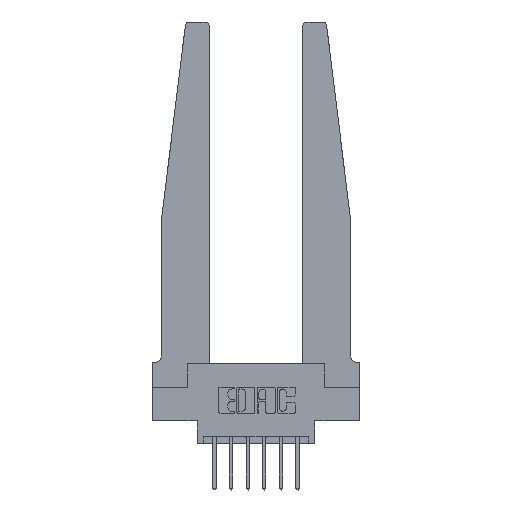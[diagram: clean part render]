
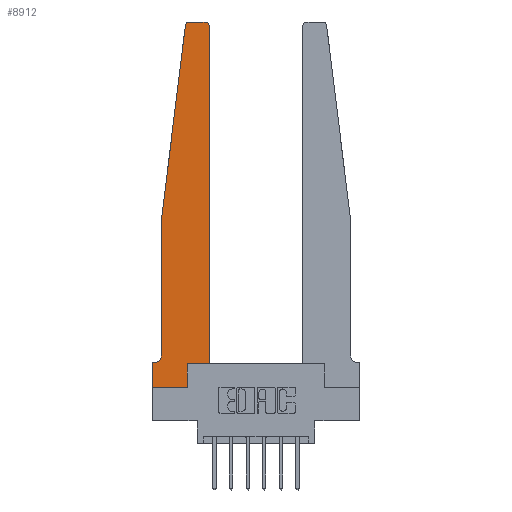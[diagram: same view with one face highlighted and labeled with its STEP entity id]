
A CAD part, top view. The second image highlights one B-rep face of the part: STEP entity #8912.
In plain terms, the highlighted planar face has unit normal (0, 0, 1).
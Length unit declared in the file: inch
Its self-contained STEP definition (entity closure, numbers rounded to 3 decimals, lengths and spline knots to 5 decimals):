
#233 = CARTESIAN_POINT ( 'NONE',  ( 0.27653, 2.72, 0.37 ) ) ;
#350 = AXIS2_PLACEMENT_3D ( 'NONE', #6943, #617, #8035 ) ;
#370 = ORIENTED_EDGE ( 'NONE', *, *, #1534, .T. ) ;
#470 = DIRECTION ( 'NONE',  ( 1., 0., 0. ) ) ;
#531 = VECTOR ( 'NONE', #470, 39.37008 ) ;
#533 = VERTEX_POINT ( 'NONE', #2530 ) ;
#617 = DIRECTION ( 'NONE',  ( 0., 0., 1. ) ) ;
#885 = LINE ( 'NONE', #7896, #531 ) ;
#1322 = DIRECTION ( 'NONE',  ( 1., 0., 0. ) ) ;
#1493 = VECTOR ( 'NONE', #3000, 39.37008 ) ;
#1534 = EDGE_CURVE ( 'NONE', #13502, #2419, #11196, .T. ) ;
#1874 = LINE ( 'NONE', #3142, #2214 ) ;
#1982 = CARTESIAN_POINT ( 'NONE',  ( 0.065, 1.25, 0.37 ) ) ;
#2042 = VERTEX_POINT ( 'NONE', #1982 ) ;
#2214 = VECTOR ( 'NONE', #5263, 39.37008 ) ;
#2419 = VERTEX_POINT ( 'NONE', #2809 ) ;
#2530 = CARTESIAN_POINT ( 'NONE',  ( 0., 0., 0.37 ) ) ;
#2577 = ORIENTED_EDGE ( 'NONE', *, *, #4362, .T. ) ;
#2700 = EDGE_CURVE ( 'NONE', #8825, #11561, #4251, .T. ) ;
#2713 = CARTESIAN_POINT ( 'NONE',  ( 0., 0., 0.37 ) ) ;
#2779 = ORIENTED_EDGE ( 'NONE', *, *, #11386, .T. ) ;
#2809 = CARTESIAN_POINT ( 'NONE',  ( 0.425, 2.72, 0.37 ) ) ;
#3000 = DIRECTION ( 'NONE',  ( 0., -1., 0. ) ) ;
#3011 = VECTOR ( 'NONE', #9632, 39.37008 ) ;
#3061 = ORIENTED_EDGE ( 'NONE', *, *, #11150, .T. ) ;
#3142 = CARTESIAN_POINT ( 'NONE',  ( 0.25, 2.75, 0.37 ) ) ;
#3811 = CARTESIAN_POINT ( 'NONE',  ( 0.2605, 0.18, 0.37 ) ) ;
#3930 = CARTESIAN_POINT ( 'NONE',  ( 0.395, 2.75, 0.37 ) ) ;
#4018 = EDGE_CURVE ( 'NONE', #4080, #13502, #885, .T. ) ;
#4080 = VERTEX_POINT ( 'NONE', #3811 ) ;
#4125 = FACE_OUTER_BOUND ( 'NONE', #7262, .T. ) ;
#4251 = CIRCLE ( 'NONE', #10601, 0.05 ) ;
#4277 = DIRECTION ( 'NONE',  ( 0., 1., 0. ) ) ;
#4280 = DIRECTION ( 'NONE',  ( -1., 0., 0. ) ) ;
#4308 = ORIENTED_EDGE ( 'NONE', *, *, #7747, .T. ) ;
#4355 = LINE ( 'NONE', #12104, #12741 ) ;
#4362 = EDGE_CURVE ( 'NONE', #4863, #12184, #1874, .T. ) ;
#4521 = DIRECTION ( 'NONE',  ( 0., 0., -1. ) ) ;
#4762 = DIRECTION ( 'NONE',  ( 0., 1., 0. ) ) ;
#4863 = VERTEX_POINT ( 'NONE', #3930 ) ;
#5131 = VECTOR ( 'NONE', #11581, 39.37008 ) ;
#5263 = DIRECTION ( 'NONE',  ( -1., 0., 0. ) ) ;
#5359 = EDGE_CURVE ( 'NONE', #5531, #4080, #4355, .T. ) ;
#5436 = CARTESIAN_POINT ( 'NONE',  ( 0.395, 2.72, 0.37 ) ) ;
#5531 = VERTEX_POINT ( 'NONE', #10488 ) ;
#5604 = CIRCLE ( 'NONE', #5686, 0.03 ) ;
#5686 = AXIS2_PLACEMENT_3D ( 'NONE', #233, #7655, #1322 ) ;
#5702 = CARTESIAN_POINT ( 'NONE',  ( 0.015, 0.1875, 0.37 ) ) ;
#6032 = EDGE_CURVE ( 'NONE', #2042, #8825, #13206, .T. ) ;
#6205 = EDGE_CURVE ( 'NONE', #533, #5531, #13701, .T. ) ;
#6461 = DIRECTION ( 'NONE',  ( 1., 0., 0. ) ) ;
#6476 = EDGE_CURVE ( 'NONE', #9056, #2042, #10756, .T. ) ;
#6810 = CARTESIAN_POINT ( 'NONE',  ( 0.065, 0.2375, 0.37 ) ) ;
#6943 = CARTESIAN_POINT ( 'NONE',  ( 0., 0.1875, 0.37 ) ) ;
#7046 = EDGE_CURVE ( 'NONE', #11561, #13651, #10402, .T. ) ;
#7102 = LINE ( 'NONE', #13484, #1493 ) ;
#7262 = EDGE_LOOP ( 'NONE', ( #2577, #4308, #10296, #10727, #11767, #8503, #3061, #11403, #12300, #12495, #370, #2779 ) ) ;
#7509 = CARTESIAN_POINT ( 'NONE',  ( 0.065, 1.25, 0.37 ) ) ;
#7655 = DIRECTION ( 'NONE',  ( 0., 0., 1. ) ) ;
#7747 = EDGE_CURVE ( 'NONE', #12184, #9056, #5604, .T. ) ;
#7896 = CARTESIAN_POINT ( 'NONE',  ( 0.425, 0.18, 0.37 ) ) ;
#7972 = DIRECTION ( 'NONE',  ( 1., 0., 0. ) ) ;
#8035 = DIRECTION ( 'NONE',  ( 1., 0., 0. ) ) ;
#8503 = ORIENTED_EDGE ( 'NONE', *, *, #7046, .T. ) ;
#8825 = VERTEX_POINT ( 'NONE', #6810 ) ;
#8905 = CARTESIAN_POINT ( 'NONE',  ( 0.27653, 2.75, 0.37 ) ) ;
#8912 = ADVANCED_FACE ( 'NONE', ( #4125 ), #9043, .T. ) ;
#9043 = PLANE ( 'NONE',  #350 ) ;
#9056 = VERTEX_POINT ( 'NONE', #12449 ) ;
#9171 = AXIS2_PLACEMENT_3D ( 'NONE', #5436, #12795, #6461 ) ;
#9632 = DIRECTION ( 'NONE',  ( 0., -1., 0. ) ) ;
#10076 = CIRCLE ( 'NONE', #9171, 0.03 ) ;
#10296 = ORIENTED_EDGE ( 'NONE', *, *, #6476, .T. ) ;
#10402 = LINE ( 'NONE', #12682, #12865 ) ;
#10488 = CARTESIAN_POINT ( 'NONE',  ( 0.2605, 0., 0.37 ) ) ;
#10507 = CARTESIAN_POINT ( 'NONE',  ( 0.065, 1.25, 0.37 ) ) ;
#10575 = CARTESIAN_POINT ( 'NONE',  ( 0.425, 0.18, 0.37 ) ) ;
#10601 = AXIS2_PLACEMENT_3D ( 'NONE', #10843, #4521, #11903 ) ;
#10727 = ORIENTED_EDGE ( 'NONE', *, *, #6032, .T. ) ;
#10756 = LINE ( 'NONE', #10507, #5131 ) ;
#10843 = CARTESIAN_POINT ( 'NONE',  ( 0.015, 0.2375, 0.37 ) ) ;
#11150 = EDGE_CURVE ( 'NONE', #13651, #533, #7102, .T. ) ;
#11196 = LINE ( 'NONE', #10575, #11543 ) ;
#11386 = EDGE_CURVE ( 'NONE', #2419, #4863, #10076, .T. ) ;
#11403 = ORIENTED_EDGE ( 'NONE', *, *, #6205, .T. ) ;
#11543 = VECTOR ( 'NONE', #4277, 39.37008 ) ;
#11561 = VERTEX_POINT ( 'NONE', #5702 ) ;
#11581 = DIRECTION ( 'NONE',  ( -0.122, -0.992, 0. ) ) ;
#11767 = ORIENTED_EDGE ( 'NONE', *, *, #2700, .T. ) ;
#11903 = DIRECTION ( 'NONE',  ( -1., 0., 0. ) ) ;
#12104 = CARTESIAN_POINT ( 'NONE',  ( 0.2605, 0.18, 0.37 ) ) ;
#12184 = VERTEX_POINT ( 'NONE', #8905 ) ;
#12300 = ORIENTED_EDGE ( 'NONE', *, *, #5359, .T. ) ;
#12449 = CARTESIAN_POINT ( 'NONE',  ( 0.24675, 2.72367, 0.37 ) ) ;
#12495 = ORIENTED_EDGE ( 'NONE', *, *, #4018, .T. ) ;
#12635 = CARTESIAN_POINT ( 'NONE',  ( 0., 0.1875, 0.37 ) ) ;
#12682 = CARTESIAN_POINT ( 'NONE',  ( 0.065, 0.1875, 0.37 ) ) ;
#12741 = VECTOR ( 'NONE', #4762, 39.37008 ) ;
#12795 = DIRECTION ( 'NONE',  ( 0., 0., 1. ) ) ;
#12865 = VECTOR ( 'NONE', #4280, 39.37008 ) ;
#13206 = LINE ( 'NONE', #7509, #3011 ) ;
#13326 = CARTESIAN_POINT ( 'NONE',  ( 0.425, 0.18, 0.37 ) ) ;
#13369 = VECTOR ( 'NONE', #7972, 39.37008 ) ;
#13484 = CARTESIAN_POINT ( 'NONE',  ( 0., 0., 0.37 ) ) ;
#13502 = VERTEX_POINT ( 'NONE', #13326 ) ;
#13651 = VERTEX_POINT ( 'NONE', #12635 ) ;
#13701 = LINE ( 'NONE', #2713, #13369 ) ;
